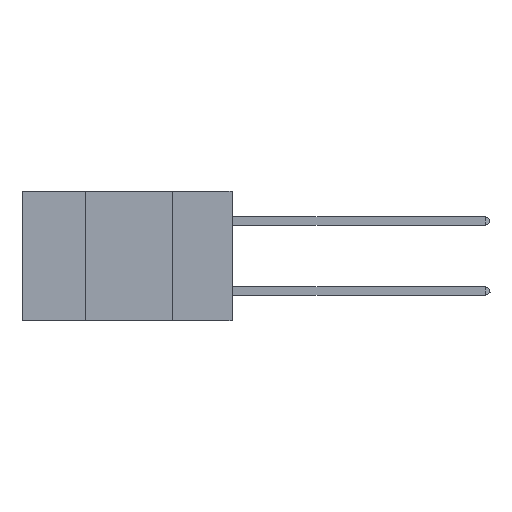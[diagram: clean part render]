
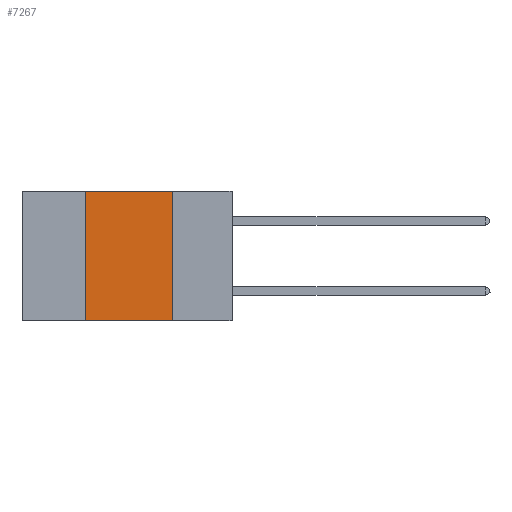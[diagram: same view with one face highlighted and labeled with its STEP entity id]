
A CAD part, left-side view. The second image highlights one B-rep face of the part: STEP entity #7267.
In plain terms, the highlighted planar face has unit normal (-1, 0, 0).
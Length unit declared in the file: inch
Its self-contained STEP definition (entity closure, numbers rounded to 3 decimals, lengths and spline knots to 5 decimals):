
#709 = LINE ( 'NONE', #9874, #2665 ) ;
#754 = CARTESIAN_POINT ( 'NONE',  ( 0., 0.6, -0.37 ) ) ;
#915 = VECTOR ( 'NONE', #9960, 39.37008 ) ;
#1688 = DIRECTION ( 'NONE',  ( 0., 0., -1. ) ) ;
#1995 = DIRECTION ( 'NONE',  ( 1., 0., 0. ) ) ;
#2086 = EDGE_LOOP ( 'NONE', ( #4394, #6814, #18083, #16352 ) ) ;
#2606 = LINE ( 'NONE', #18674, #915 ) ;
#2665 = VECTOR ( 'NONE', #6896, 39.37008 ) ;
#2837 = VERTEX_POINT ( 'NONE', #21981 ) ;
#2985 = VERTEX_POINT ( 'NONE', #17627 ) ;
#4394 = ORIENTED_EDGE ( 'NONE', *, *, #18041, .F. ) ;
#4870 = EDGE_CURVE ( 'NONE', #2837, #2985, #709, .T. ) ;
#5111 = CARTESIAN_POINT ( 'NONE',  ( 0., 0.17, 0. ) ) ;
#6112 = EDGE_CURVE ( 'NONE', #2837, #14926, #15216, .T. ) ;
#6814 = ORIENTED_EDGE ( 'NONE', *, *, #21455, .F. ) ;
#6896 = DIRECTION ( 'NONE',  ( 0., 0., 1. ) ) ;
#7267 = ADVANCED_FACE ( 'NONE', ( #19336 ), #9090, .F. ) ;
#7806 = DIRECTION ( 'NONE',  ( 0., -1., 0. ) ) ;
#8095 = LINE ( 'NONE', #5111, #8871 ) ;
#8871 = VECTOR ( 'NONE', #20921, 39.37008 ) ;
#9044 = CARTESIAN_POINT ( 'NONE',  ( 0., 0.17, -0.37 ) ) ;
#9090 = PLANE ( 'NONE',  #14509 ) ;
#9874 = CARTESIAN_POINT ( 'NONE',  ( 0., 0.42, 0. ) ) ;
#9960 = DIRECTION ( 'NONE',  ( 0., -1., 0. ) ) ;
#14091 = VECTOR ( 'NONE', #7806, 39.37008 ) ;
#14509 = AXIS2_PLACEMENT_3D ( 'NONE', #16941, #1995, #1688 ) ;
#14926 = VERTEX_POINT ( 'NONE', #9044 ) ;
#15216 = LINE ( 'NONE', #754, #14091 ) ;
#16352 = ORIENTED_EDGE ( 'NONE', *, *, #6112, .T. ) ;
#16941 = CARTESIAN_POINT ( 'NONE',  ( 0., 0.6, 0. ) ) ;
#17627 = CARTESIAN_POINT ( 'NONE',  ( 0., 0.42, 0. ) ) ;
#18041 = EDGE_CURVE ( 'NONE', #21322, #14926, #8095, .T. ) ;
#18083 = ORIENTED_EDGE ( 'NONE', *, *, #4870, .F. ) ;
#18674 = CARTESIAN_POINT ( 'NONE',  ( 0., 0.6, 0. ) ) ;
#19336 = FACE_OUTER_BOUND ( 'NONE', #2086, .T. ) ;
#20921 = DIRECTION ( 'NONE',  ( 0., 0., -1. ) ) ;
#21322 = VERTEX_POINT ( 'NONE', #21846 ) ;
#21455 = EDGE_CURVE ( 'NONE', #2985, #21322, #2606, .T. ) ;
#21846 = CARTESIAN_POINT ( 'NONE',  ( 0., 0.17, 0. ) ) ;
#21981 = CARTESIAN_POINT ( 'NONE',  ( 0., 0.42, -0.37 ) ) ;
